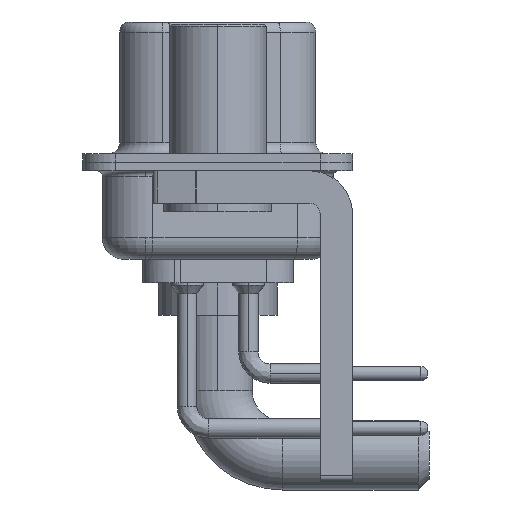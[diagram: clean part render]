
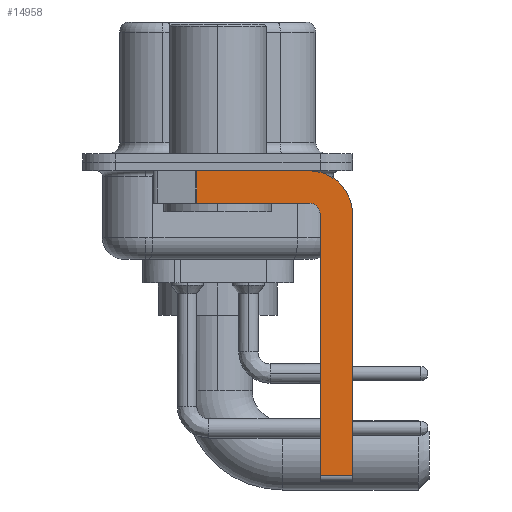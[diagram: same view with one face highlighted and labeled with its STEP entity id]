
A CAD part, left-side view. The second image highlights one B-rep face of the part: STEP entity #14958.
In plain terms, the highlighted planar face has unit normal (-1, 0, 0).
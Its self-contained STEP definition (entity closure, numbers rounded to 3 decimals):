
#266 = EDGE_CURVE ( 'NONE', #25567, #5042, #2993, .T. ) ;
#1351 = CARTESIAN_POINT ( 'NONE',  ( -2.9, -4.25, -1.9 ) ) ;
#1491 = VECTOR ( 'NONE', #16625, 1000. ) ;
#1500 = FACE_OUTER_BOUND ( 'NONE', #17898, .T. ) ;
#1551 = CARTESIAN_POINT ( 'NONE',  ( -2.9, -4.25, -2.4 ) ) ;
#1742 = LINE ( 'NONE', #25876, #15767 ) ;
#2246 = EDGE_CURVE ( 'NONE', #25567, #24970, #9200, .T. ) ;
#2602 = ORIENTED_EDGE ( 'NONE', *, *, #14772, .F. ) ;
#2993 = LINE ( 'NONE', #20531, #1491 ) ;
#3107 = VERTEX_POINT ( 'NONE', #3680 ) ;
#3148 = VECTOR ( 'NONE', #15781, 1000. ) ;
#3239 = ORIENTED_EDGE ( 'NONE', *, *, #15129, .F. ) ;
#3241 = DIRECTION ( 'NONE',  ( 0., 0., -1. ) ) ;
#3680 = CARTESIAN_POINT ( 'NONE',  ( -2.9, -4.25, -1.9 ) ) ;
#4704 = EDGE_CURVE ( 'NONE', #25092, #4864, #4979, .T. ) ;
#4864 = VERTEX_POINT ( 'NONE', #16455 ) ;
#4979 = LINE ( 'NONE', #9598, #18378 ) ;
#5042 = VERTEX_POINT ( 'NONE', #21492 ) ;
#5102 = CARTESIAN_POINT ( 'NONE',  ( -2.9, -4.25, -0.4 ) ) ;
#5405 = VECTOR ( 'NONE', #10147, 1000. ) ;
#5733 = VERTEX_POINT ( 'NONE', #14096 ) ;
#7151 = EDGE_CURVE ( 'NONE', #8189, #5733, #26811, .T. ) ;
#7893 = EDGE_CURVE ( 'NONE', #5042, #3107, #22248, .T. ) ;
#8189 = VERTEX_POINT ( 'NONE', #5102 ) ;
#8512 = CARTESIAN_POINT ( 'NONE',  ( -2.9, -6.25, -14.55 ) ) ;
#8709 = CARTESIAN_POINT ( 'NONE',  ( -2.9, 3., -0.4 ) ) ;
#8722 = AXIS2_PLACEMENT_3D ( 'NONE', #12294, #22923, #3241 ) ;
#9200 = LINE ( 'NONE', #27133, #3148 ) ;
#9598 = CARTESIAN_POINT ( 'NONE',  ( -2.9, 0.978, -1.9 ) ) ;
#10041 = DIRECTION ( 'NONE',  ( 0., 0., 1. ) ) ;
#10147 = DIRECTION ( 'NONE',  ( 0., 1., 0. ) ) ;
#10512 = ORIENTED_EDGE ( 'NONE', *, *, #7893, .F. ) ;
#10672 = DIRECTION ( 'NONE',  ( 0., 0., -1. ) ) ;
#11474 = ORIENTED_EDGE ( 'NONE', *, *, #2246, .T. ) ;
#12030 = CARTESIAN_POINT ( 'NONE',  ( -2.9, -4.75, -14.55 ) ) ;
#12173 = CARTESIAN_POINT ( 'NONE',  ( -2.9, -4.25, -2.4 ) ) ;
#12294 = CARTESIAN_POINT ( 'NONE',  ( -2.9, -4.25, -2.4 ) ) ;
#14096 = CARTESIAN_POINT ( 'NONE',  ( -2.9, -6.25, -2.4 ) ) ;
#14242 = CARTESIAN_POINT ( 'NONE',  ( -2.9, 0.978, -0.4 ) ) ;
#14714 = LINE ( 'NONE', #1351, #5405 ) ;
#14772 = EDGE_CURVE ( 'NONE', #3107, #4864, #14714, .T. ) ;
#14958 = ADVANCED_FACE ( 'NONE', ( #1500 ), #21334, .F. ) ;
#15129 = EDGE_CURVE ( 'NONE', #25092, #8189, #17587, .T. ) ;
#15767 = VECTOR ( 'NONE', #10672, 1000. ) ;
#15781 = DIRECTION ( 'NONE',  ( 0., -1., 0. ) ) ;
#16310 = ORIENTED_EDGE ( 'NONE', *, *, #4704, .T. ) ;
#16455 = CARTESIAN_POINT ( 'NONE',  ( -2.9, 0.978, -1.9 ) ) ;
#16625 = DIRECTION ( 'NONE',  ( 0., 0., 1. ) ) ;
#16787 = DIRECTION ( 'NONE',  ( 0., 0., -1. ) ) ;
#17404 = VECTOR ( 'NONE', #19317, 1000. ) ;
#17587 = LINE ( 'NONE', #8709, #17404 ) ;
#17898 = EDGE_LOOP ( 'NONE', ( #3239, #16310, #2602, #10512, #22883, #11474, #19745, #25702 ) ) ;
#18073 = AXIS2_PLACEMENT_3D ( 'NONE', #1551, #21390, #16787 ) ;
#18320 = DIRECTION ( 'NONE',  ( 0., 0., -1. ) ) ;
#18378 = VECTOR ( 'NONE', #18320, 1000. ) ;
#19317 = DIRECTION ( 'NONE',  ( 0., -1., 0. ) ) ;
#19745 = ORIENTED_EDGE ( 'NONE', *, *, #24893, .F. ) ;
#20531 = CARTESIAN_POINT ( 'NONE',  ( -2.9, -4.75, -14.8 ) ) ;
#21334 = PLANE ( 'NONE',  #8722 ) ;
#21390 = DIRECTION ( 'NONE',  ( 1., 0., 0. ) ) ;
#21492 = CARTESIAN_POINT ( 'NONE',  ( -2.9, -4.75, -2.4 ) ) ;
#22248 = CIRCLE ( 'NONE', #25019, 0.5 ) ;
#22883 = ORIENTED_EDGE ( 'NONE', *, *, #266, .F. ) ;
#22923 = DIRECTION ( 'NONE',  ( 1., 0., 0. ) ) ;
#24893 = EDGE_CURVE ( 'NONE', #5733, #24970, #1742, .T. ) ;
#24970 = VERTEX_POINT ( 'NONE', #8512 ) ;
#25019 = AXIS2_PLACEMENT_3D ( 'NONE', #12173, #25242, #10041 ) ;
#25092 = VERTEX_POINT ( 'NONE', #14242 ) ;
#25242 = DIRECTION ( 'NONE',  ( -1., 0., 0. ) ) ;
#25567 = VERTEX_POINT ( 'NONE', #12030 ) ;
#25702 = ORIENTED_EDGE ( 'NONE', *, *, #7151, .F. ) ;
#25876 = CARTESIAN_POINT ( 'NONE',  ( -2.9, -6.25, -2.4 ) ) ;
#26811 = CIRCLE ( 'NONE', #18073, 2. ) ;
#27133 = CARTESIAN_POINT ( 'NONE',  ( -2.9, -4.25, -14.55 ) ) ;
